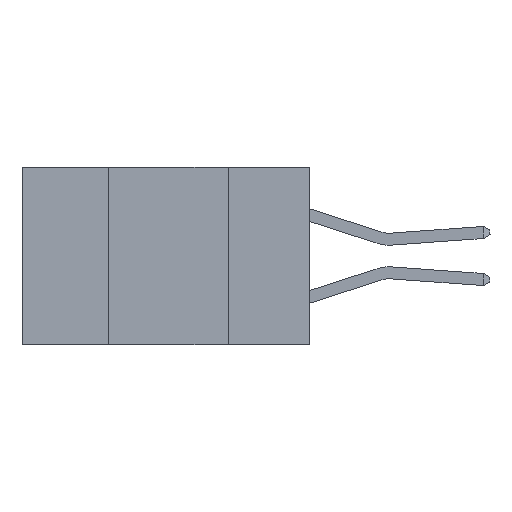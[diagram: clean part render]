
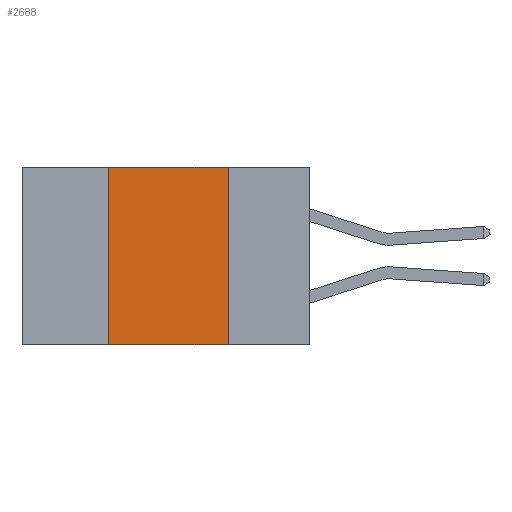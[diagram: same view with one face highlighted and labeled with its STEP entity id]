
A CAD part, left-side view. The second image highlights one B-rep face of the part: STEP entity #2688.
In plain terms, the highlighted planar face has unit normal (-1, 0, 0).
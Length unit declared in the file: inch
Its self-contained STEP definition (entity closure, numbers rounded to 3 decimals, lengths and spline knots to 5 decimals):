
#99 = CARTESIAN_POINT ( 'NONE',  ( 0., 0.17, -0.37 ) ) ;
#217 = CARTESIAN_POINT ( 'NONE',  ( 0., 0.6, -0.37 ) ) ;
#882 = CARTESIAN_POINT ( 'NONE',  ( 0., 0.42, -0.37 ) ) ;
#961 = VECTOR ( 'NONE', #5246, 39.37008 ) ;
#1197 = VERTEX_POINT ( 'NONE', #8985 ) ;
#1304 = AXIS2_PLACEMENT_3D ( 'NONE', #3283, #6702, #4119 ) ;
#1413 = ORIENTED_EDGE ( 'NONE', *, *, #3272, .F. ) ;
#1684 = CARTESIAN_POINT ( 'NONE',  ( 0., 0.6, 0. ) ) ;
#2019 = CARTESIAN_POINT ( 'NONE',  ( 0., 0.17, -0.37 ) ) ;
#2034 = EDGE_LOOP ( 'NONE', ( #10880, #3326, #1413, #10273 ) ) ;
#2278 = EDGE_CURVE ( 'NONE', #9632, #1197, #5809, .T. ) ;
#2688 = ADVANCED_FACE ( 'NONE', ( #10159 ), #10821, .F. ) ;
#2733 = DIRECTION ( 'NONE',  ( 0., -1., 0. ) ) ;
#3181 = VERTEX_POINT ( 'NONE', #3197 ) ;
#3197 = CARTESIAN_POINT ( 'NONE',  ( 0., 0.42, -0.37 ) ) ;
#3272 = EDGE_CURVE ( 'NONE', #3181, #9632, #6948, .T. ) ;
#3283 = CARTESIAN_POINT ( 'NONE',  ( 0., 0.6, 0. ) ) ;
#3326 = ORIENTED_EDGE ( 'NONE', *, *, #2278, .F. ) ;
#4119 = DIRECTION ( 'NONE',  ( 0., 0., -1. ) ) ;
#4237 = VERTEX_POINT ( 'NONE', #99 ) ;
#5240 = VECTOR ( 'NONE', #8070, 39.37008 ) ;
#5246 = DIRECTION ( 'NONE',  ( 0., -1., 0. ) ) ;
#5303 = DIRECTION ( 'NONE',  ( 0., 0., 1. ) ) ;
#5568 = EDGE_CURVE ( 'NONE', #1197, #4237, #8804, .T. ) ;
#5809 = LINE ( 'NONE', #1684, #6644 ) ;
#5814 = VECTOR ( 'NONE', #5303, 39.37008 ) ;
#5861 = CARTESIAN_POINT ( 'NONE',  ( 0., 0.42, 0. ) ) ;
#6644 = VECTOR ( 'NONE', #2733, 39.37008 ) ;
#6702 = DIRECTION ( 'NONE',  ( 1., 0., 0. ) ) ;
#6948 = LINE ( 'NONE', #882, #5814 ) ;
#7931 = LINE ( 'NONE', #217, #961 ) ;
#8070 = DIRECTION ( 'NONE',  ( 0., 0., -1. ) ) ;
#8516 = EDGE_CURVE ( 'NONE', #3181, #4237, #7931, .T. ) ;
#8804 = LINE ( 'NONE', #2019, #5240 ) ;
#8985 = CARTESIAN_POINT ( 'NONE',  ( 0., 0.17, 0. ) ) ;
#9632 = VERTEX_POINT ( 'NONE', #5861 ) ;
#10159 = FACE_OUTER_BOUND ( 'NONE', #2034, .T. ) ;
#10273 = ORIENTED_EDGE ( 'NONE', *, *, #8516, .T. ) ;
#10821 = PLANE ( 'NONE',  #1304 ) ;
#10880 = ORIENTED_EDGE ( 'NONE', *, *, #5568, .F. ) ;
